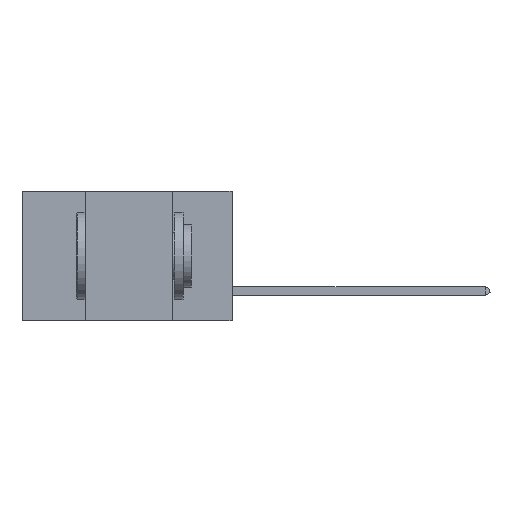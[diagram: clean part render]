
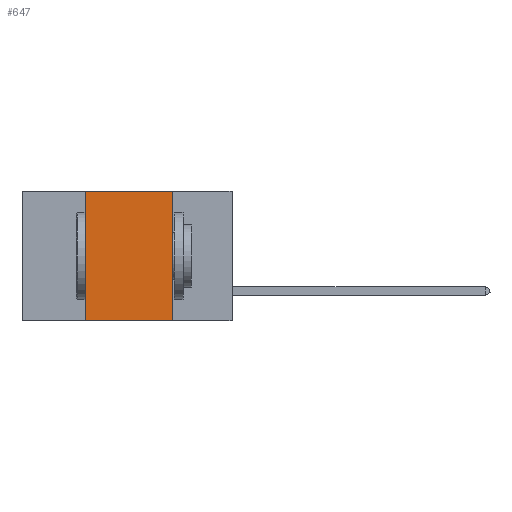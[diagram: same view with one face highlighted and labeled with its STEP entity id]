
A CAD part, left-side view. The second image highlights one B-rep face of the part: STEP entity #647.
In plain terms, the highlighted planar face has unit normal (-1, 0, 0).
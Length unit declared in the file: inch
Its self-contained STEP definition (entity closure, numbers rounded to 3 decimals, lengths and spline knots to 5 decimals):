
#56 = CARTESIAN_POINT ( 'NONE',  ( 0., 0.6, -0.37 ) ) ;
#586 = VECTOR ( 'NONE', #6014, 39.37008 ) ;
#647 = ADVANCED_FACE ( 'NONE', ( #14816 ), #933, .F. ) ;
#774 = VERTEX_POINT ( 'NONE', #10824 ) ;
#916 = CARTESIAN_POINT ( 'NONE',  ( 0., 0.42, 0. ) ) ;
#933 = PLANE ( 'NONE',  #8585 ) ;
#1141 = LINE ( 'NONE', #916, #14635 ) ;
#1753 = VERTEX_POINT ( 'NONE', #14165 ) ;
#3486 = DIRECTION ( 'NONE',  ( 0., 0., -1. ) ) ;
#3659 = ORIENTED_EDGE ( 'NONE', *, *, #6521, .T. ) ;
#4040 = VERTEX_POINT ( 'NONE', #7309 ) ;
#4600 = DIRECTION ( 'NONE',  ( 0., -1., 0. ) ) ;
#5389 = DIRECTION ( 'NONE',  ( 0., 0., -1. ) ) ;
#5860 = VECTOR ( 'NONE', #5389, 39.37008 ) ;
#6014 = DIRECTION ( 'NONE',  ( 0., -1., 0. ) ) ;
#6521 = EDGE_CURVE ( 'NONE', #774, #1753, #7981, .T. ) ;
#6563 = EDGE_CURVE ( 'NONE', #13409, #4040, #17324, .T. ) ;
#7309 = CARTESIAN_POINT ( 'NONE',  ( 0., 0.17, 0. ) ) ;
#7535 = VECTOR ( 'NONE', #4600, 39.37008 ) ;
#7981 = LINE ( 'NONE', #56, #7535 ) ;
#8571 = CARTESIAN_POINT ( 'NONE',  ( 0., 0.42, 0. ) ) ;
#8585 = AXIS2_PLACEMENT_3D ( 'NONE', #10512, #14743, #3486 ) ;
#9143 = ORIENTED_EDGE ( 'NONE', *, *, #11956, .F. ) ;
#9514 = LINE ( 'NONE', #12363, #5860 ) ;
#10349 = ORIENTED_EDGE ( 'NONE', *, *, #15614, .F. ) ;
#10512 = CARTESIAN_POINT ( 'NONE',  ( 0., 0.6, 0. ) ) ;
#10824 = CARTESIAN_POINT ( 'NONE',  ( 0., 0.42, -0.37 ) ) ;
#11399 = CARTESIAN_POINT ( 'NONE',  ( 0., 0.6, 0. ) ) ;
#11834 = ORIENTED_EDGE ( 'NONE', *, *, #6563, .F. ) ;
#11956 = EDGE_CURVE ( 'NONE', #4040, #1753, #9514, .T. ) ;
#12339 = EDGE_LOOP ( 'NONE', ( #9143, #11834, #10349, #3659 ) ) ;
#12363 = CARTESIAN_POINT ( 'NONE',  ( 0., 0.17, 0. ) ) ;
#13409 = VERTEX_POINT ( 'NONE', #8571 ) ;
#14165 = CARTESIAN_POINT ( 'NONE',  ( 0., 0.17, -0.37 ) ) ;
#14635 = VECTOR ( 'NONE', #17383, 39.37008 ) ;
#14743 = DIRECTION ( 'NONE',  ( 1., 0., 0. ) ) ;
#14816 = FACE_OUTER_BOUND ( 'NONE', #12339, .T. ) ;
#15614 = EDGE_CURVE ( 'NONE', #774, #13409, #1141, .T. ) ;
#17324 = LINE ( 'NONE', #11399, #586 ) ;
#17383 = DIRECTION ( 'NONE',  ( 0., 0., 1. ) ) ;
